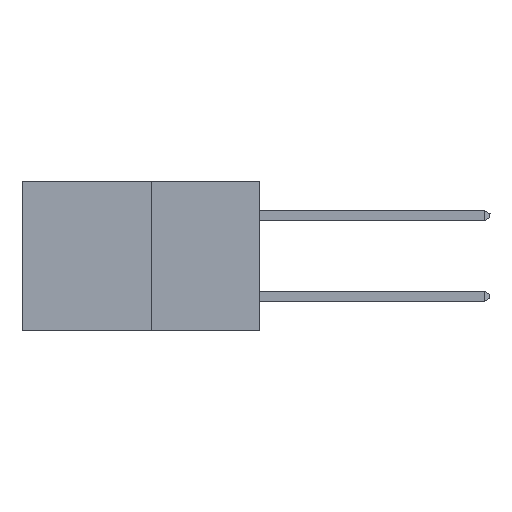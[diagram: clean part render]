
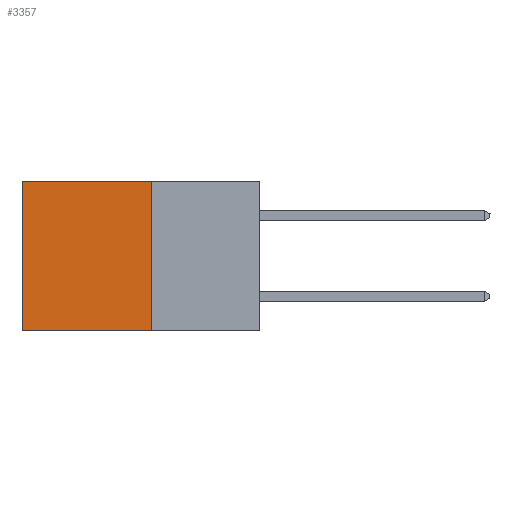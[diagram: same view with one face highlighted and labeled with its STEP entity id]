
A CAD part, left-side view. The second image highlights one B-rep face of the part: STEP entity #3357.
In plain terms, the highlighted planar face has unit normal (-1, 0, 0).
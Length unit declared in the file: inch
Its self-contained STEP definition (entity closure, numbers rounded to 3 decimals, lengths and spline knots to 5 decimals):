
#218 = EDGE_CURVE ( 'NONE', #9603, #5574, #3487, .T. ) ;
#502 = ORIENTED_EDGE ( 'NONE', *, *, #9816, .T. ) ;
#556 = CARTESIAN_POINT ( 'NONE',  ( 0.277, 0.27, -0.37 ) ) ;
#602 = EDGE_LOOP ( 'NONE', ( #5594, #3214, #1552, #502 ) ) ;
#802 = CARTESIAN_POINT ( 'NONE',  ( 0.277, 0.59, -0.37 ) ) ;
#1042 = LINE ( 'NONE', #802, #7231 ) ;
#1552 = ORIENTED_EDGE ( 'NONE', *, *, #218, .F. ) ;
#2756 = DIRECTION ( 'NONE',  ( 1., 0., 0. ) ) ;
#3043 = DIRECTION ( 'NONE',  ( 0., 1., 0. ) ) ;
#3162 = EDGE_CURVE ( 'NONE', #5574, #7190, #9770, .T. ) ;
#3214 = ORIENTED_EDGE ( 'NONE', *, *, #3162, .F. ) ;
#3357 = ADVANCED_FACE ( 'NONE', ( #9655 ), #9278, .F. ) ;
#3487 = LINE ( 'NONE', #556, #9495 ) ;
#3630 = DIRECTION ( 'NONE',  ( 0., 1., 0. ) ) ;
#3666 = CARTESIAN_POINT ( 'NONE',  ( 0.277, 0.27, 0. ) ) ;
#3919 = VERTEX_POINT ( 'NONE', #5534 ) ;
#4965 = VECTOR ( 'NONE', #3630, 39.37008 ) ;
#5098 = CARTESIAN_POINT ( 'NONE',  ( 0.277, 0.59, -0.37 ) ) ;
#5433 = DIRECTION ( 'NONE',  ( 0., 0., -1. ) ) ;
#5534 = CARTESIAN_POINT ( 'NONE',  ( 0.277, 0.59, 0. ) ) ;
#5574 = VERTEX_POINT ( 'NONE', #6696 ) ;
#5594 = ORIENTED_EDGE ( 'NONE', *, *, #7968, .T. ) ;
#5775 = VECTOR ( 'NONE', #3043, 39.37008 ) ;
#6696 = CARTESIAN_POINT ( 'NONE',  ( 0.277, 0.27, -0.37 ) ) ;
#6759 = CARTESIAN_POINT ( 'NONE',  ( 0.277, 0.27, 0. ) ) ;
#6786 = DIRECTION ( 'NONE',  ( 0., 0., -1. ) ) ;
#7190 = VERTEX_POINT ( 'NONE', #5098 ) ;
#7231 = VECTOR ( 'NONE', #6786, 39.37008 ) ;
#7348 = AXIS2_PLACEMENT_3D ( 'NONE', #9947, #2756, #5433 ) ;
#7968 = EDGE_CURVE ( 'NONE', #3919, #7190, #1042, .T. ) ;
#8086 = DIRECTION ( 'NONE',  ( 0., 0., -1. ) ) ;
#8866 = CARTESIAN_POINT ( 'NONE',  ( 0.277, 0.27, -0.37 ) ) ;
#9278 = PLANE ( 'NONE',  #7348 ) ;
#9309 = LINE ( 'NONE', #3666, #4965 ) ;
#9495 = VECTOR ( 'NONE', #8086, 39.37008 ) ;
#9603 = VERTEX_POINT ( 'NONE', #6759 ) ;
#9655 = FACE_OUTER_BOUND ( 'NONE', #602, .T. ) ;
#9770 = LINE ( 'NONE', #8866, #5775 ) ;
#9816 = EDGE_CURVE ( 'NONE', #9603, #3919, #9309, .T. ) ;
#9947 = CARTESIAN_POINT ( 'NONE',  ( 0.277, 0.27, -0.37 ) ) ;
